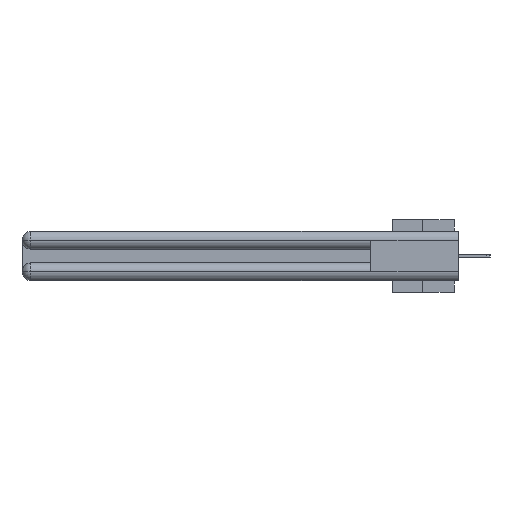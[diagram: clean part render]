
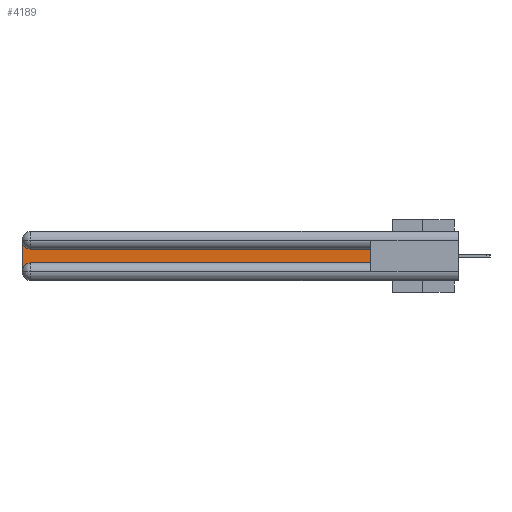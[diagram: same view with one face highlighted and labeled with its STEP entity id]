
A CAD part, left-side view. The second image highlights one B-rep face of the part: STEP entity #4189.
In plain terms, the highlighted planar face has unit normal (-1, 0, 0).
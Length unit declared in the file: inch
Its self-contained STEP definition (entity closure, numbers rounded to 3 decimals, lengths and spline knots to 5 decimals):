
#262 = VERTEX_POINT ( 'NONE', #22357 ) ;
#940 = CARTESIAN_POINT ( 'NONE',  ( 0.075, 0.6, -0.1225 ) ) ;
#1588 = DIRECTION ( 'NONE',  ( 0., 0., -1. ) ) ;
#2562 = VERTEX_POINT ( 'NONE', #26786 ) ;
#3436 = ORIENTED_EDGE ( 'NONE', *, *, #18876, .T. ) ;
#4189 = ADVANCED_FACE ( 'NONE', ( #20459 ), #19823, .F. ) ;
#4263 = VECTOR ( 'NONE', #9755, 39.37008 ) ;
#5266 = DIRECTION ( 'NONE',  ( 0., 0., -1. ) ) ;
#6069 = LINE ( 'NONE', #15471, #4263 ) ;
#6436 = EDGE_LOOP ( 'NONE', ( #29845, #24866, #17995, #3436, #12090, #27586 ) ) ;
#7490 = CARTESIAN_POINT ( 'NONE',  ( 0.075, 2.94, -0.2775 ) ) ;
#9213 = CIRCLE ( 'NONE', #11655, 0.06 ) ;
#9755 = DIRECTION ( 'NONE',  ( 0., 1., 0. ) ) ;
#10427 = DIRECTION ( 'NONE',  ( 0., 0., -1. ) ) ;
#10467 = VECTOR ( 'NONE', #32856, 39.37008 ) ;
#10809 = LINE ( 'NONE', #36246, #14876 ) ;
#11099 = DIRECTION ( 'NONE',  ( 0., -1., 0. ) ) ;
#11655 = AXIS2_PLACEMENT_3D ( 'NONE', #7490, #27861, #10427 ) ;
#12090 = ORIENTED_EDGE ( 'NONE', *, *, #37314, .T. ) ;
#12323 = VERTEX_POINT ( 'NONE', #28386 ) ;
#14876 = VECTOR ( 'NONE', #15910, 39.37008 ) ;
#15471 = CARTESIAN_POINT ( 'NONE',  ( 0.075, 0.6, -0.1225 ) ) ;
#15910 = DIRECTION ( 'NONE',  ( 0., 0., 1. ) ) ;
#17295 = VERTEX_POINT ( 'NONE', #940 ) ;
#17624 = CARTESIAN_POINT ( 'NONE',  ( 0.075, 3., -0.2775 ) ) ;
#17995 = ORIENTED_EDGE ( 'NONE', *, *, #27362, .T. ) ;
#18876 = EDGE_CURVE ( 'NONE', #33872, #262, #9213, .T. ) ;
#19068 = DIRECTION ( 'NONE',  ( 1., 0., 0. ) ) ;
#19823 = PLANE ( 'NONE',  #20291 ) ;
#19937 = CIRCLE ( 'NONE', #35491, 0.06 ) ;
#20059 = LINE ( 'NONE', #21193, #10467 ) ;
#20291 = AXIS2_PLACEMENT_3D ( 'NONE', #25538, #22778, #5266 ) ;
#20459 = FACE_OUTER_BOUND ( 'NONE', #6436, .T. ) ;
#21193 = CARTESIAN_POINT ( 'NONE',  ( 0.075, 3., -0.2175 ) ) ;
#22357 = CARTESIAN_POINT ( 'NONE',  ( 0.075, 2.94, -0.2175 ) ) ;
#22778 = DIRECTION ( 'NONE',  ( 1., 0., 0. ) ) ;
#24268 = EDGE_CURVE ( 'NONE', #17295, #12323, #6069, .T. ) ;
#24866 = ORIENTED_EDGE ( 'NONE', *, *, #37747, .T. ) ;
#25538 = CARTESIAN_POINT ( 'NONE',  ( 0.075, 3., -0.1225 ) ) ;
#25546 = CARTESIAN_POINT ( 'NONE',  ( 0.075, 0.6, -0.2175 ) ) ;
#25615 = CARTESIAN_POINT ( 'NONE',  ( 0.075, 0.6, -0.2175 ) ) ;
#26786 = CARTESIAN_POINT ( 'NONE',  ( 0.075, 3., -0.0625 ) ) ;
#27362 = EDGE_CURVE ( 'NONE', #2562, #33872, #20059, .T. ) ;
#27586 = ORIENTED_EDGE ( 'NONE', *, *, #34596, .T. ) ;
#27861 = DIRECTION ( 'NONE',  ( 1., 0., 0. ) ) ;
#28386 = CARTESIAN_POINT ( 'NONE',  ( 0.075, 2.94, -0.1225 ) ) ;
#29512 = LINE ( 'NONE', #25615, #35413 ) ;
#29845 = ORIENTED_EDGE ( 'NONE', *, *, #24268, .T. ) ;
#32856 = DIRECTION ( 'NONE',  ( 0., 0., -1. ) ) ;
#33872 = VERTEX_POINT ( 'NONE', #17624 ) ;
#34596 = EDGE_CURVE ( 'NONE', #35462, #17295, #10809, .T. ) ;
#35413 = VECTOR ( 'NONE', #11099, 39.37008 ) ;
#35462 = VERTEX_POINT ( 'NONE', #25546 ) ;
#35491 = AXIS2_PLACEMENT_3D ( 'NONE', #36470, #19068, #1588 ) ;
#36246 = CARTESIAN_POINT ( 'NONE',  ( 0.075, 0.6, -0.2175 ) ) ;
#36470 = CARTESIAN_POINT ( 'NONE',  ( 0.075, 2.94, -0.0625 ) ) ;
#37314 = EDGE_CURVE ( 'NONE', #262, #35462, #29512, .T. ) ;
#37747 = EDGE_CURVE ( 'NONE', #12323, #2562, #19937, .T. ) ;
